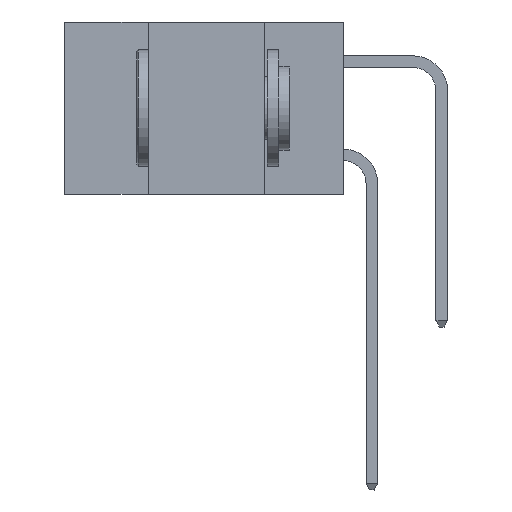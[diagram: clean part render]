
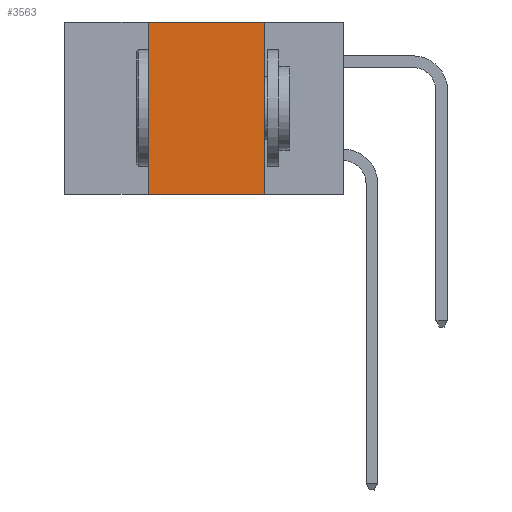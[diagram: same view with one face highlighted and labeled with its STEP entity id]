
A CAD part, left-side view. The second image highlights one B-rep face of the part: STEP entity #3563.
In plain terms, the highlighted planar face has unit normal (-1, 0, 0).
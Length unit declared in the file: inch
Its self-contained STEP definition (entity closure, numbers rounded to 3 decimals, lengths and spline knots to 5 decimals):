
#805 = EDGE_CURVE ( 'NONE', #13313, #18259, #31388, .T. ) ;
#1941 = CARTESIAN_POINT ( 'NONE',  ( 0., 0.6, -0.37 ) ) ;
#2828 = CARTESIAN_POINT ( 'NONE',  ( 0., 0.6, 0. ) ) ;
#2947 = DIRECTION ( 'NONE',  ( 0., 0., -1. ) ) ;
#3563 = ADVANCED_FACE ( 'NONE', ( #30324 ), #13916, .F. ) ;
#4574 = DIRECTION ( 'NONE',  ( 0., -1., 0. ) ) ;
#5567 = CARTESIAN_POINT ( 'NONE',  ( 0., 0.17, -0.37 ) ) ;
#8373 = LINE ( 'NONE', #1941, #14701 ) ;
#10596 = CARTESIAN_POINT ( 'NONE',  ( 0., 0.6, 0. ) ) ;
#10856 = ORIENTED_EDGE ( 'NONE', *, *, #32670, .F. ) ;
#11450 = VERTEX_POINT ( 'NONE', #5567 ) ;
#13187 = CARTESIAN_POINT ( 'NONE',  ( 0., 0.42, 0. ) ) ;
#13313 = VERTEX_POINT ( 'NONE', #15997 ) ;
#13869 = DIRECTION ( 'NONE',  ( 1., 0., 0. ) ) ;
#13916 = PLANE ( 'NONE',  #17958 ) ;
#14073 = CARTESIAN_POINT ( 'NONE',  ( 0., 0.17, 0. ) ) ;
#14701 = VECTOR ( 'NONE', #18110, 39.37008 ) ;
#15997 = CARTESIAN_POINT ( 'NONE',  ( 0., 0.42, 0. ) ) ;
#16765 = DIRECTION ( 'NONE',  ( 0., 0., -1. ) ) ;
#16968 = VERTEX_POINT ( 'NONE', #23936 ) ;
#17462 = EDGE_LOOP ( 'NONE', ( #10856, #19807, #20318, #23817 ) ) ;
#17958 = AXIS2_PLACEMENT_3D ( 'NONE', #10596, #13869, #2947 ) ;
#18110 = DIRECTION ( 'NONE',  ( 0., -1., 0. ) ) ;
#18259 = VERTEX_POINT ( 'NONE', #21833 ) ;
#19807 = ORIENTED_EDGE ( 'NONE', *, *, #805, .F. ) ;
#20318 = ORIENTED_EDGE ( 'NONE', *, *, #29098, .F. ) ;
#20353 = EDGE_CURVE ( 'NONE', #16968, #11450, #8373, .T. ) ;
#20473 = VECTOR ( 'NONE', #34279, 39.37008 ) ;
#21833 = CARTESIAN_POINT ( 'NONE',  ( 0., 0.17, 0. ) ) ;
#23575 = VECTOR ( 'NONE', #4574, 39.37008 ) ;
#23817 = ORIENTED_EDGE ( 'NONE', *, *, #20353, .T. ) ;
#23936 = CARTESIAN_POINT ( 'NONE',  ( 0., 0.42, -0.37 ) ) ;
#27274 = LINE ( 'NONE', #14073, #33421 ) ;
#28244 = LINE ( 'NONE', #13187, #20473 ) ;
#29098 = EDGE_CURVE ( 'NONE', #16968, #13313, #28244, .T. ) ;
#30324 = FACE_OUTER_BOUND ( 'NONE', #17462, .T. ) ;
#31388 = LINE ( 'NONE', #2828, #23575 ) ;
#32670 = EDGE_CURVE ( 'NONE', #18259, #11450, #27274, .T. ) ;
#33421 = VECTOR ( 'NONE', #16765, 39.37008 ) ;
#34279 = DIRECTION ( 'NONE',  ( 0., 0., 1. ) ) ;
